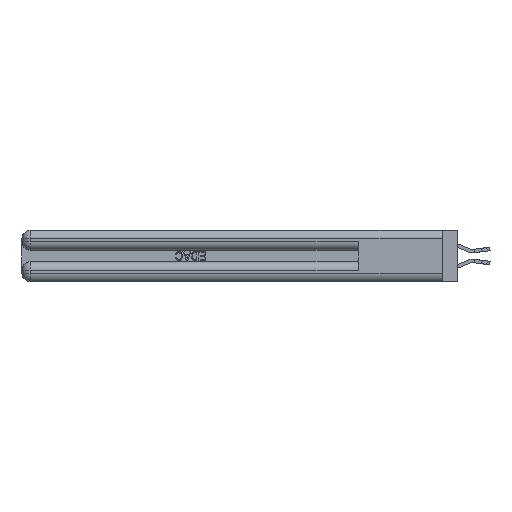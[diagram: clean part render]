
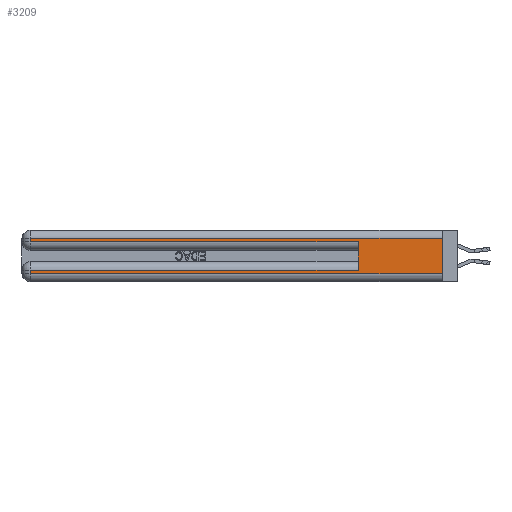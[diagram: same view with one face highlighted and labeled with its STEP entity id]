
A CAD part, left-side view. The second image highlights one B-rep face of the part: STEP entity #3209.
In plain terms, the highlighted planar face has unit normal (-1, 0, 0).
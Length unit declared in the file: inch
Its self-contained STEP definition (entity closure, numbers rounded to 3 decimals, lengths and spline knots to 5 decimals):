
#719 = DIRECTION ( 'NONE',  ( 0., 0., -1. ) ) ;
#742 = VERTEX_POINT ( 'NONE', #37017 ) ;
#828 = LINE ( 'NONE', #19699, #15830 ) ;
#1578 = CARTESIAN_POINT ( 'NONE',  ( 0., 0., 0.31 ) ) ;
#1761 = DIRECTION ( 'NONE',  ( 0., 1., 0. ) ) ;
#2420 = VERTEX_POINT ( 'NONE', #3798 ) ;
#2507 = VECTOR ( 'NONE', #14186, 39.37008 ) ;
#3209 = ADVANCED_FACE ( 'NONE', ( #18632 ), #9615, .F. ) ;
#3798 = CARTESIAN_POINT ( 'NONE',  ( 0., 2.94, 0.285 ) ) ;
#4220 = DIRECTION ( 'NONE',  ( 0., -1., 0. ) ) ;
#4749 = EDGE_CURVE ( 'NONE', #19409, #742, #32064, .T. ) ;
#5085 = ORIENTED_EDGE ( 'NONE', *, *, #33883, .T. ) ;
#5224 = EDGE_CURVE ( 'NONE', #2420, #9574, #31089, .T. ) ;
#8000 = VECTOR ( 'NONE', #4220, 39.37008 ) ;
#8141 = CARTESIAN_POINT ( 'NONE',  ( 0., 0., 0.31 ) ) ;
#8251 = VECTOR ( 'NONE', #1761, 39.37008 ) ;
#8719 = VECTOR ( 'NONE', #32409, 39.37008 ) ;
#9574 = VERTEX_POINT ( 'NONE', #17529 ) ;
#9615 = PLANE ( 'NONE',  #20451 ) ;
#9653 = LINE ( 'NONE', #11563, #8719 ) ;
#10248 = CARTESIAN_POINT ( 'NONE',  ( 0., 0.6, 0.085 ) ) ;
#10738 = CARTESIAN_POINT ( 'NONE',  ( 0., 2.94, 0.06 ) ) ;
#10763 = ORIENTED_EDGE ( 'NONE', *, *, #10797, .T. ) ;
#10797 = EDGE_CURVE ( 'NONE', #742, #25499, #9653, .T. ) ;
#11563 = CARTESIAN_POINT ( 'NONE',  ( 0., 2.94, 0.37 ) ) ;
#12603 = EDGE_CURVE ( 'NONE', #16385, #33974, #26370, .T. ) ;
#14186 = DIRECTION ( 'NONE',  ( 0., 1., 0. ) ) ;
#14696 = LINE ( 'NONE', #20587, #28683 ) ;
#15830 = VECTOR ( 'NONE', #22705, 39.37008 ) ;
#15967 = LINE ( 'NONE', #33946, #8000 ) ;
#16385 = VERTEX_POINT ( 'NONE', #1578 ) ;
#16874 = EDGE_CURVE ( 'NONE', #25499, #24275, #15967, .T. ) ;
#17129 = CARTESIAN_POINT ( 'NONE',  ( 0., 0., 0.37 ) ) ;
#17529 = CARTESIAN_POINT ( 'NONE',  ( 0., 0.6, 0.285 ) ) ;
#18632 = FACE_OUTER_BOUND ( 'NONE', #33666, .T. ) ;
#18672 = DIRECTION ( 'NONE',  ( 1., 0., 0. ) ) ;
#19229 = CARTESIAN_POINT ( 'NONE',  ( 0., 0., 0.06 ) ) ;
#19409 = VERTEX_POINT ( 'NONE', #10248 ) ;
#19699 = CARTESIAN_POINT ( 'NONE',  ( 0., 2.94, 0.37 ) ) ;
#20402 = LINE ( 'NONE', #17129, #28281 ) ;
#20451 = AXIS2_PLACEMENT_3D ( 'NONE', #36468, #18672, #719 ) ;
#20587 = CARTESIAN_POINT ( 'NONE',  ( 0., 0.6, 0.145 ) ) ;
#20609 = ORIENTED_EDGE ( 'NONE', *, *, #4749, .T. ) ;
#22606 = ORIENTED_EDGE ( 'NONE', *, *, #16874, .T. ) ;
#22698 = ORIENTED_EDGE ( 'NONE', *, *, #12603, .T. ) ;
#22705 = DIRECTION ( 'NONE',  ( 0., 0., -1. ) ) ;
#22762 = CARTESIAN_POINT ( 'NONE',  ( 0., 0., 0.085 ) ) ;
#23816 = ORIENTED_EDGE ( 'NONE', *, *, #5224, .T. ) ;
#23874 = EDGE_CURVE ( 'NONE', #19409, #9574, #14696, .T. ) ;
#24045 = ORIENTED_EDGE ( 'NONE', *, *, #23874, .F. ) ;
#24275 = VERTEX_POINT ( 'NONE', #19229 ) ;
#25330 = DIRECTION ( 'NONE',  ( 0., -1., 0. ) ) ;
#25499 = VERTEX_POINT ( 'NONE', #10738 ) ;
#26370 = LINE ( 'NONE', #8141, #2507 ) ;
#28281 = VECTOR ( 'NONE', #32101, 39.37008 ) ;
#28683 = VECTOR ( 'NONE', #35364, 39.37008 ) ;
#30153 = VECTOR ( 'NONE', #25330, 39.37008 ) ;
#31089 = LINE ( 'NONE', #34131, #30153 ) ;
#31206 = ORIENTED_EDGE ( 'NONE', *, *, #34740, .F. ) ;
#32064 = LINE ( 'NONE', #22762, #8251 ) ;
#32101 = DIRECTION ( 'NONE',  ( 0., 0., -1. ) ) ;
#32409 = DIRECTION ( 'NONE',  ( 0., 0., -1. ) ) ;
#33666 = EDGE_LOOP ( 'NONE', ( #31206, #22698, #5085, #23816, #24045, #20609, #10763, #22606 ) ) ;
#33883 = EDGE_CURVE ( 'NONE', #33974, #2420, #828, .T. ) ;
#33946 = CARTESIAN_POINT ( 'NONE',  ( 0., 0., 0.06 ) ) ;
#33974 = VERTEX_POINT ( 'NONE', #37830 ) ;
#34131 = CARTESIAN_POINT ( 'NONE',  ( 0., 0., 0.285 ) ) ;
#34740 = EDGE_CURVE ( 'NONE', #16385, #24275, #20402, .T. ) ;
#35364 = DIRECTION ( 'NONE',  ( 0., 0., 1. ) ) ;
#36468 = CARTESIAN_POINT ( 'NONE',  ( 0., 0., 0.37 ) ) ;
#37017 = CARTESIAN_POINT ( 'NONE',  ( 0., 2.94, 0.085 ) ) ;
#37830 = CARTESIAN_POINT ( 'NONE',  ( 0., 2.94, 0.31 ) ) ;
